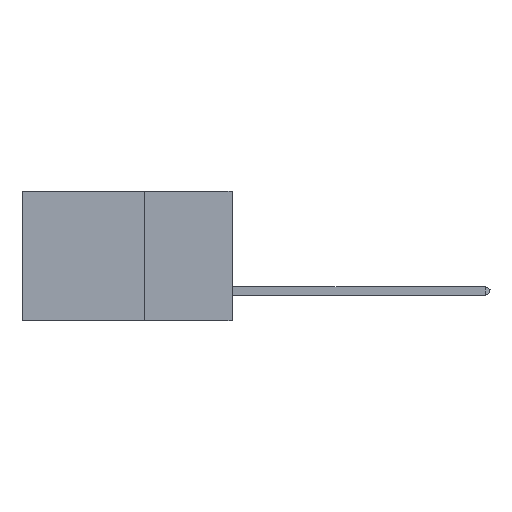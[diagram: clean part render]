
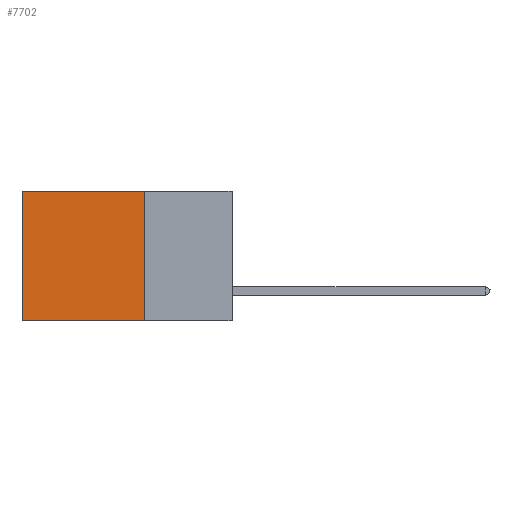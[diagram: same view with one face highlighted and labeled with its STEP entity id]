
A CAD part, left-side view. The second image highlights one B-rep face of the part: STEP entity #7702.
In plain terms, the highlighted planar face has unit normal (-1, 0, 0).
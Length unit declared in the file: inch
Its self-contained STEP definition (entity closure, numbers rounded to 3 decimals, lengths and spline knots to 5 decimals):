
#816 = DIRECTION ( 'NONE',  ( 1., 0., 0. ) ) ;
#862 = CARTESIAN_POINT ( 'NONE',  ( 0.2875, 0.25, -0.37 ) ) ;
#2334 = CARTESIAN_POINT ( 'NONE',  ( 0.2875, 0.25, 0. ) ) ;
#4150 = EDGE_LOOP ( 'NONE', ( #4423, #5649, #23982, #6003 ) ) ;
#4423 = ORIENTED_EDGE ( 'NONE', *, *, #15209, .T. ) ;
#5649 = ORIENTED_EDGE ( 'NONE', *, *, #17601, .F. ) ;
#6003 = ORIENTED_EDGE ( 'NONE', *, *, #7755, .T. ) ;
#6013 = LINE ( 'NONE', #28149, #23241 ) ;
#7702 = ADVANCED_FACE ( 'NONE', ( #25111 ), #35573, .F. ) ;
#7755 = EDGE_CURVE ( 'NONE', #10939, #15361, #27236, .T. ) ;
#7884 = VECTOR ( 'NONE', #35302, 39.37008 ) ;
#10939 = VERTEX_POINT ( 'NONE', #18533 ) ;
#11148 = AXIS2_PLACEMENT_3D ( 'NONE', #24202, #816, #35053 ) ;
#13298 = CARTESIAN_POINT ( 'NONE',  ( 0.2875, 0.25, 0. ) ) ;
#14794 = LINE ( 'NONE', #2334, #28541 ) ;
#15209 = EDGE_CURVE ( 'NONE', #15361, #24593, #6013, .T. ) ;
#15361 = VERTEX_POINT ( 'NONE', #25906 ) ;
#16005 = CARTESIAN_POINT ( 'NONE',  ( 0.2875, 0.25, -0.37 ) ) ;
#17601 = EDGE_CURVE ( 'NONE', #32868, #24593, #33061, .T. ) ;
#18533 = CARTESIAN_POINT ( 'NONE',  ( 0.2875, 0.25, 0. ) ) ;
#21241 = EDGE_CURVE ( 'NONE', #10939, #32868, #14794, .T. ) ;
#21381 = CARTESIAN_POINT ( 'NONE',  ( 0.2875, 0.6, -0.37 ) ) ;
#21446 = VECTOR ( 'NONE', #24032, 39.37008 ) ;
#23241 = VECTOR ( 'NONE', #28387, 39.37008 ) ;
#23982 = ORIENTED_EDGE ( 'NONE', *, *, #21241, .F. ) ;
#24032 = DIRECTION ( 'NONE',  ( 0., 1., 0. ) ) ;
#24202 = CARTESIAN_POINT ( 'NONE',  ( 0.2875, 0.25, 0. ) ) ;
#24356 = DIRECTION ( 'NONE',  ( 0., 0., -1. ) ) ;
#24593 = VERTEX_POINT ( 'NONE', #21381 ) ;
#25111 = FACE_OUTER_BOUND ( 'NONE', #4150, .T. ) ;
#25906 = CARTESIAN_POINT ( 'NONE',  ( 0.2875, 0.6, 0. ) ) ;
#27236 = LINE ( 'NONE', #13298, #7884 ) ;
#28149 = CARTESIAN_POINT ( 'NONE',  ( 0.2875, 0.6, 0. ) ) ;
#28387 = DIRECTION ( 'NONE',  ( 0., 0., -1. ) ) ;
#28541 = VECTOR ( 'NONE', #24356, 39.37008 ) ;
#32868 = VERTEX_POINT ( 'NONE', #862 ) ;
#33061 = LINE ( 'NONE', #16005, #21446 ) ;
#35053 = DIRECTION ( 'NONE',  ( 0., 0., -1. ) ) ;
#35302 = DIRECTION ( 'NONE',  ( 0., 1., 0. ) ) ;
#35573 = PLANE ( 'NONE',  #11148 ) ;
